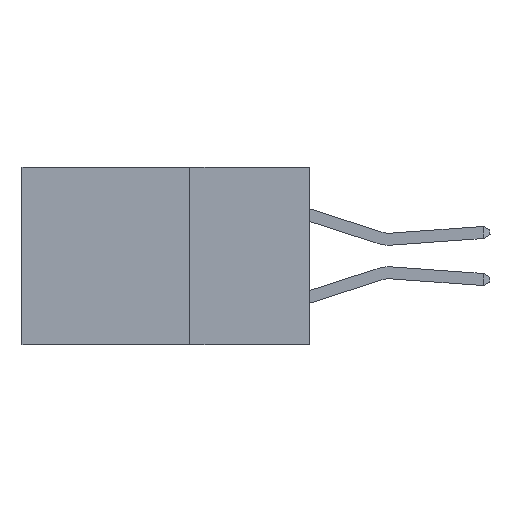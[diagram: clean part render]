
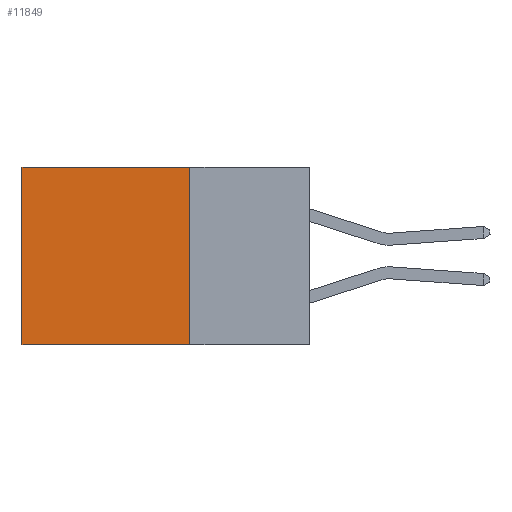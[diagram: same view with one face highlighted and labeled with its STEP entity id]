
A CAD part, left-side view. The second image highlights one B-rep face of the part: STEP entity #11849.
In plain terms, the highlighted planar face has unit normal (-1, 0, 0).
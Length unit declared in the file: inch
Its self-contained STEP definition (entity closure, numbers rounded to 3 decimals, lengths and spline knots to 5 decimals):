
#265 = ORIENTED_EDGE ( 'NONE', *, *, #19734, .F. ) ;
#847 = VECTOR ( 'NONE', #3688, 39.37008 ) ;
#1003 = ORIENTED_EDGE ( 'NONE', *, *, #22171, .T. ) ;
#1531 = CARTESIAN_POINT ( 'NONE',  ( 0.2615, 0.6, 0. ) ) ;
#1643 = EDGE_CURVE ( 'NONE', #8063, #9703, #17580, .T. ) ;
#3672 = VERTEX_POINT ( 'NONE', #4409 ) ;
#3688 = DIRECTION ( 'NONE',  ( 0., 0., -1. ) ) ;
#3769 = EDGE_LOOP ( 'NONE', ( #23072, #19552, #265, #1003 ) ) ;
#4409 = CARTESIAN_POINT ( 'NONE',  ( 0.2615, 0.25, 0. ) ) ;
#8063 = VERTEX_POINT ( 'NONE', #21405 ) ;
#8303 = CARTESIAN_POINT ( 'NONE',  ( 0.2615, 0.6, -0.37 ) ) ;
#9703 = VERTEX_POINT ( 'NONE', #8303 ) ;
#9939 = VERTEX_POINT ( 'NONE', #1531 ) ;
#11242 = PLANE ( 'NONE',  #24584 ) ;
#11632 = FACE_OUTER_BOUND ( 'NONE', #3769, .T. ) ;
#11849 = ADVANCED_FACE ( 'NONE', ( #11632 ), #11242, .F. ) ;
#13258 = DIRECTION ( 'NONE',  ( 1., 0., 0. ) ) ;
#13536 = DIRECTION ( 'NONE',  ( 0., 1., 0. ) ) ;
#13792 = CARTESIAN_POINT ( 'NONE',  ( 0.2615, 0.25, -0.37 ) ) ;
#13922 = LINE ( 'NONE', #13792, #847 ) ;
#14265 = DIRECTION ( 'NONE',  ( 0., 1., 0. ) ) ;
#15326 = DIRECTION ( 'NONE',  ( 0., 0., -1. ) ) ;
#16294 = LINE ( 'NONE', #20758, #24630 ) ;
#16522 = VECTOR ( 'NONE', #15326, 39.37008 ) ;
#17580 = LINE ( 'NONE', #25819, #24333 ) ;
#19552 = ORIENTED_EDGE ( 'NONE', *, *, #1643, .F. ) ;
#19734 = EDGE_CURVE ( 'NONE', #3672, #8063, #13922, .T. ) ;
#20758 = CARTESIAN_POINT ( 'NONE',  ( 0.2615, 0.25, 0. ) ) ;
#21031 = CARTESIAN_POINT ( 'NONE',  ( 0.2615, 0.6, -0.37 ) ) ;
#21405 = CARTESIAN_POINT ( 'NONE',  ( 0.2615, 0.25, -0.37 ) ) ;
#21555 = LINE ( 'NONE', #21031, #16522 ) ;
#21887 = DIRECTION ( 'NONE',  ( 0., 0., -1. ) ) ;
#22171 = EDGE_CURVE ( 'NONE', #3672, #9939, #16294, .T. ) ;
#23072 = ORIENTED_EDGE ( 'NONE', *, *, #25212, .T. ) ;
#24333 = VECTOR ( 'NONE', #13536, 39.37008 ) ;
#24584 = AXIS2_PLACEMENT_3D ( 'NONE', #25795, #13258, #21887 ) ;
#24630 = VECTOR ( 'NONE', #14265, 39.37008 ) ;
#25212 = EDGE_CURVE ( 'NONE', #9939, #9703, #21555, .T. ) ;
#25795 = CARTESIAN_POINT ( 'NONE',  ( 0.2615, 0.25, -0.37 ) ) ;
#25819 = CARTESIAN_POINT ( 'NONE',  ( 0.2615, 0.25, -0.37 ) ) ;
